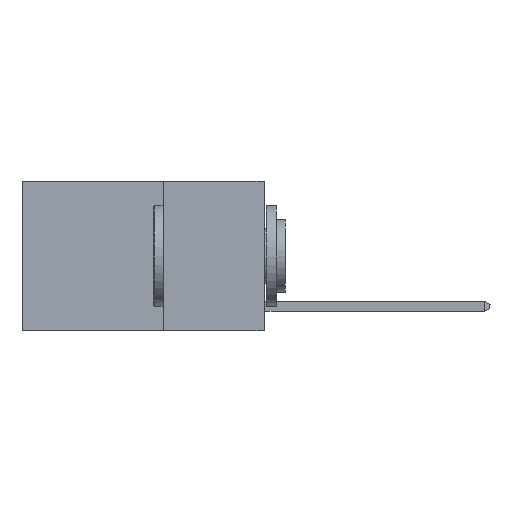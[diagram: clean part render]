
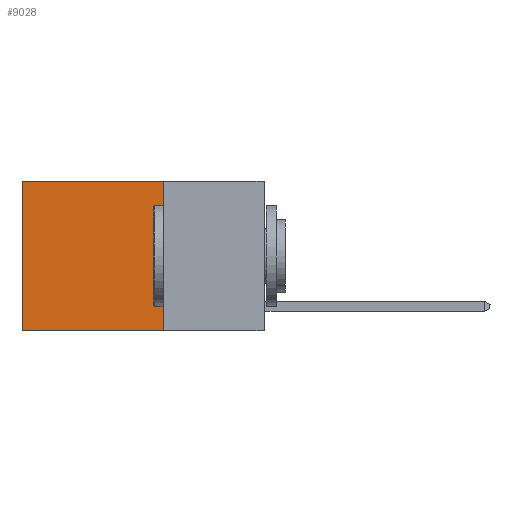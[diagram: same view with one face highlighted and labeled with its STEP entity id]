
A CAD part, left-side view. The second image highlights one B-rep face of the part: STEP entity #9028.
In plain terms, the highlighted planar face has unit normal (-1, 0, 0).
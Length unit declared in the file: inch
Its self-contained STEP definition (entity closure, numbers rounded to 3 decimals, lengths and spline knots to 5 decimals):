
#14 = DIRECTION ( 'NONE',  ( 0., 1., 0. ) ) ;
#851 = EDGE_LOOP ( 'NONE', ( #1493, #12741, #7399, #8910 ) ) ;
#989 = DIRECTION ( 'NONE',  ( 0., 1., 0. ) ) ;
#1008 = CARTESIAN_POINT ( 'NONE',  ( 0.2625, 0.25, -0.37 ) ) ;
#1045 = CARTESIAN_POINT ( 'NONE',  ( 0.2625, 0.25, 0. ) ) ;
#1493 = ORIENTED_EDGE ( 'NONE', *, *, #9118, .T. ) ;
#1813 = PLANE ( 'NONE',  #5310 ) ;
#2073 = DIRECTION ( 'NONE',  ( 0., 0., -1. ) ) ;
#2093 = VECTOR ( 'NONE', #12154, 39.37008 ) ;
#2106 = CARTESIAN_POINT ( 'NONE',  ( 0.2625, 0.6, -0.37 ) ) ;
#2533 = FACE_OUTER_BOUND ( 'NONE', #851, .T. ) ;
#2794 = DIRECTION ( 'NONE',  ( 1., 0., 0. ) ) ;
#2932 = LINE ( 'NONE', #1045, #2093 ) ;
#4051 = CARTESIAN_POINT ( 'NONE',  ( 0.2625, 0.6, 0. ) ) ;
#4227 = EDGE_CURVE ( 'NONE', #10272, #8851, #2932, .T. ) ;
#4929 = CARTESIAN_POINT ( 'NONE',  ( 0.2625, 0.25, 0. ) ) ;
#5310 = AXIS2_PLACEMENT_3D ( 'NONE', #11612, #2794, #6843 ) ;
#5596 = LINE ( 'NONE', #4929, #10695 ) ;
#6843 = DIRECTION ( 'NONE',  ( 0., 0., -1. ) ) ;
#7399 = ORIENTED_EDGE ( 'NONE', *, *, #4227, .F. ) ;
#7887 = VECTOR ( 'NONE', #2073, 39.37008 ) ;
#8351 = VERTEX_POINT ( 'NONE', #2106 ) ;
#8354 = EDGE_CURVE ( 'NONE', #8851, #8351, #11057, .T. ) ;
#8851 = VERTEX_POINT ( 'NONE', #12348 ) ;
#8910 = ORIENTED_EDGE ( 'NONE', *, *, #12811, .T. ) ;
#9028 = ADVANCED_FACE ( 'NONE', ( #2533 ), #1813, .F. ) ;
#9118 = EDGE_CURVE ( 'NONE', #11155, #8351, #11019, .T. ) ;
#10272 = VERTEX_POINT ( 'NONE', #11818 ) ;
#10695 = VECTOR ( 'NONE', #989, 39.37008 ) ;
#10914 = CARTESIAN_POINT ( 'NONE',  ( 0.2625, 0.6, 0. ) ) ;
#11019 = LINE ( 'NONE', #4051, #7887 ) ;
#11057 = LINE ( 'NONE', #1008, #12705 ) ;
#11155 = VERTEX_POINT ( 'NONE', #10914 ) ;
#11612 = CARTESIAN_POINT ( 'NONE',  ( 0.2625, 0.25, 0. ) ) ;
#11818 = CARTESIAN_POINT ( 'NONE',  ( 0.2625, 0.25, 0. ) ) ;
#12154 = DIRECTION ( 'NONE',  ( 0., 0., -1. ) ) ;
#12348 = CARTESIAN_POINT ( 'NONE',  ( 0.2625, 0.25, -0.37 ) ) ;
#12705 = VECTOR ( 'NONE', #14, 39.37008 ) ;
#12741 = ORIENTED_EDGE ( 'NONE', *, *, #8354, .F. ) ;
#12811 = EDGE_CURVE ( 'NONE', #10272, #11155, #5596, .T. ) ;
